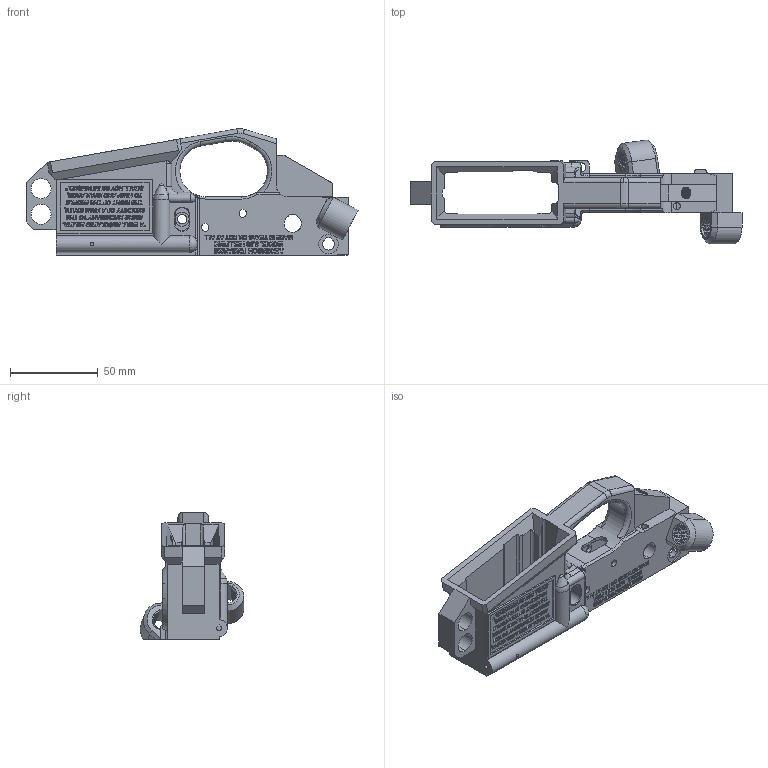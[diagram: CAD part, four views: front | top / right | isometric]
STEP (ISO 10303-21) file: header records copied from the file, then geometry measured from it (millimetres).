
FILE_DESCRIPTION (( 'STEP AP203' ), '1' );
FILE_NAME ('AF-HF-LR-PRT-NS-001-STEP.STEP', '2020-12-05T02:23:47', ( '' ), ( '' ), 'SwSTEP 2.0', 'SolidWorks 2018', '' );
FILE_SCHEMA (( 'CONFIG_CONTROL_DESIGN' ));
Products named in the file (1): AF-HF-LR-PRT-NS-001-STEP
Bounding box: 189.54 x 59.15 x 72.31 mm (x, y, z)
Volume: 98325.2 mm3; surface area: 58519.9 mm2
Topology: 1 solids, 1 shells, 3149 faces, 8627 edges, 5714 vertices
Faces by surface type: plane 2101, bspline 759, cylinder 244, torus 22, cone 19, sphere 4
Entity records: 179995 total; most frequent: CARTESIAN_POINT 106219, ORIENTED_EDGE 17242, DIRECTION 11858, EDGE_CURVE 8621, LINE 6318, VECTOR 6318, VERTEX_POINT 5713, EDGE_LOOP 3434
